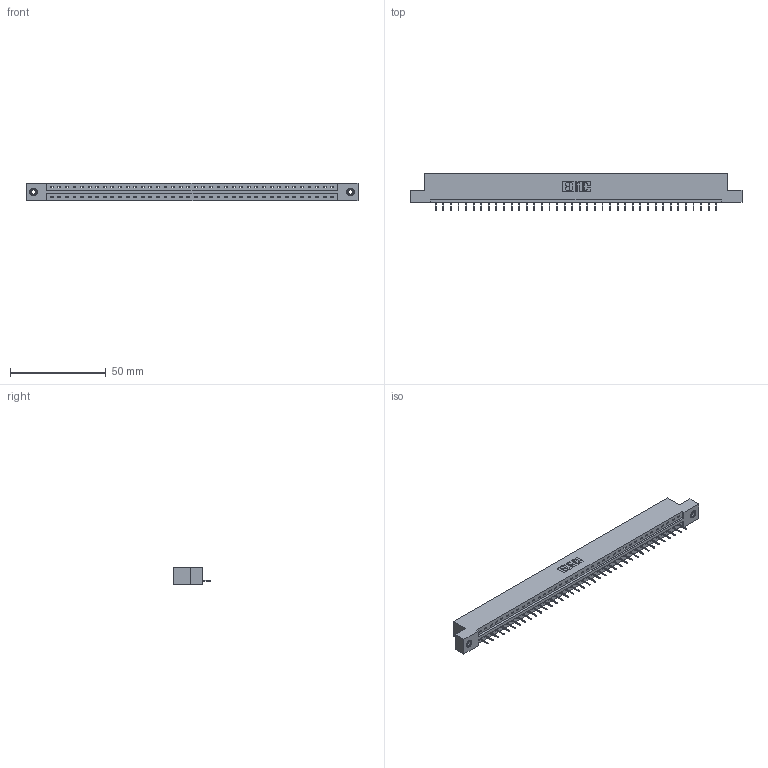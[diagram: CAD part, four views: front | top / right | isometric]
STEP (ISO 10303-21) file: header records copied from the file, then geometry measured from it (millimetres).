
FILE_DESCRIPTION (( 'STEP AP203' ), '1' );
FILE_NAME ('837-038-524-108.STEP', '2021-08-04T14:50:44', ( '' ), ( '' ), 'SwSTEP 2.0', 'SolidWorks 2020', '' );
FILE_SCHEMA (( 'CONFIG_CONTROL_DESIGN' ));
Length unit declared in the file: inch
Products named in the file (4): 345-250-001_345-250-003-102; 837-038-524-108; 345-292-001_345-293-124; 837 Part_Flush Mounting Lugs - 0.156 Dia-TI
Assembly tree (41 placements, depth 2):
  837-038-524-108
    837 Part_Flush Mounting Lugs - 0.156 Dia-TI
    345-292-001_345-293-124  x38
    345-250-001_345-250-003-102  x2
Bounding box: 173.58 x 19.69 x 9.4 mm (x, y, z)
Volume: 17834.4 mm3; surface area: 17908.9 mm2
Topology: 41 solids, 41 shells, 2682 faces, 7743 edges, 5002 vertices
Faces by surface type: plane 2078, cylinder 588, cone 12, torus 4
Entity records: 30024 total; most frequent: CARTESIAN_POINT 5207, ORIENTED_EDGE 5174, DIRECTION 4425, EDGE_CURVE 2587, LINE 2443, VECTOR 2443, VERTEX_POINT 1716, AXIS2_PLACEMENT_3D 991
